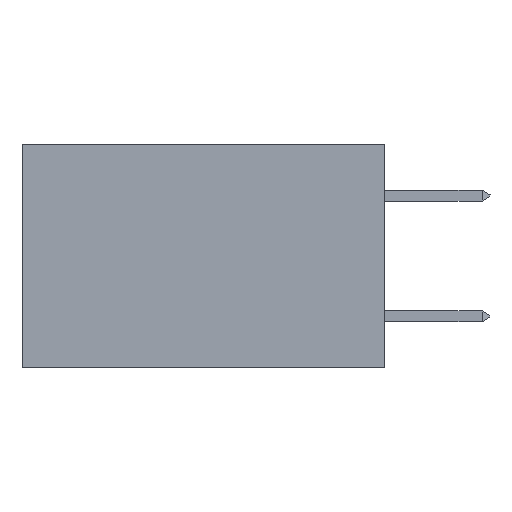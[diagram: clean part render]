
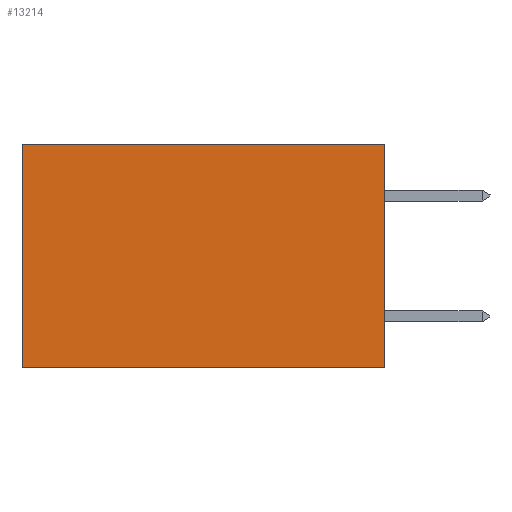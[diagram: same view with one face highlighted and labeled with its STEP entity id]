
A CAD part, left-side view. The second image highlights one B-rep face of the part: STEP entity #13214.
In plain terms, the highlighted planar face has unit normal (-1, 0, 0).
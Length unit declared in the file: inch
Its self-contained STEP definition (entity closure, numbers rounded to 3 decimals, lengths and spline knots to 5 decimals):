
#34 = VERTEX_POINT ( 'NONE', #25163 ) ;
#3200 = FACE_OUTER_BOUND ( 'NONE', #19088, .T. ) ;
#5479 = LINE ( 'NONE', #12792, #11420 ) ;
#11420 = VECTOR ( 'NONE', #36787, 39.37008 ) ;
#11737 = AXIS2_PLACEMENT_3D ( 'NONE', #38160, #41585, #21106 ) ;
#12792 = CARTESIAN_POINT ( 'NONE',  ( 0.2875, 0., 0. ) ) ;
#13214 = ADVANCED_FACE ( 'NONE', ( #3200 ), #14197, .F. ) ;
#14197 = PLANE ( 'NONE',  #11737 ) ;
#14328 = CARTESIAN_POINT ( 'NONE',  ( 0.2875, 0.6, 0. ) ) ;
#14429 = ORIENTED_EDGE ( 'NONE', *, *, #22754, .T. ) ;
#17298 = CARTESIAN_POINT ( 'NONE',  ( 0.2875, 0., -0.37 ) ) ;
#18071 = VERTEX_POINT ( 'NONE', #17298 ) ;
#18511 = DIRECTION ( 'NONE',  ( 0., 1., 0. ) ) ;
#19088 = EDGE_LOOP ( 'NONE', ( #14429, #20604, #43176, #20125 ) ) ;
#20125 = ORIENTED_EDGE ( 'NONE', *, *, #36435, .T. ) ;
#20604 = ORIENTED_EDGE ( 'NONE', *, *, #42462, .F. ) ;
#21106 = DIRECTION ( 'NONE',  ( 0., 0., -1. ) ) ;
#22368 = VERTEX_POINT ( 'NONE', #14328 ) ;
#22754 = EDGE_CURVE ( 'NONE', #22368, #35080, #29390, .T. ) ;
#23186 = CARTESIAN_POINT ( 'NONE',  ( 0.2875, 0.6, 0. ) ) ;
#24140 = DIRECTION ( 'NONE',  ( 0., 0., -1. ) ) ;
#25163 = CARTESIAN_POINT ( 'NONE',  ( 0.2875, 0., 0. ) ) ;
#26028 = LINE ( 'NONE', #41145, #44177 ) ;
#26629 = DIRECTION ( 'NONE',  ( 0., 0., -1. ) ) ;
#28343 = VECTOR ( 'NONE', #18511, 39.37008 ) ;
#29390 = LINE ( 'NONE', #23186, #35294 ) ;
#31945 = EDGE_CURVE ( 'NONE', #34, #18071, #26028, .T. ) ;
#35080 = VERTEX_POINT ( 'NONE', #43432 ) ;
#35294 = VECTOR ( 'NONE', #26629, 39.37008 ) ;
#35568 = CARTESIAN_POINT ( 'NONE',  ( 0.2875, 0., -0.37 ) ) ;
#36435 = EDGE_CURVE ( 'NONE', #34, #22368, #5479, .T. ) ;
#36787 = DIRECTION ( 'NONE',  ( 0., 1., 0. ) ) ;
#37466 = LINE ( 'NONE', #35568, #28343 ) ;
#38160 = CARTESIAN_POINT ( 'NONE',  ( 0.2875, 0., 0. ) ) ;
#41145 = CARTESIAN_POINT ( 'NONE',  ( 0.2875, 0., 0. ) ) ;
#41585 = DIRECTION ( 'NONE',  ( 1., 0., 0. ) ) ;
#42462 = EDGE_CURVE ( 'NONE', #18071, #35080, #37466, .T. ) ;
#43176 = ORIENTED_EDGE ( 'NONE', *, *, #31945, .F. ) ;
#43432 = CARTESIAN_POINT ( 'NONE',  ( 0.2875, 0.6, -0.37 ) ) ;
#44177 = VECTOR ( 'NONE', #24140, 39.37008 ) ;
